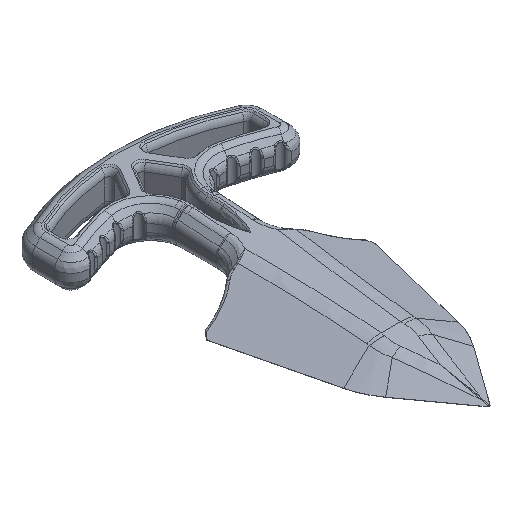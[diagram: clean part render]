
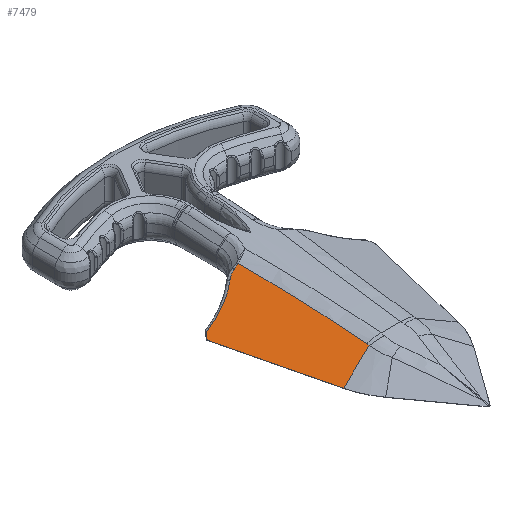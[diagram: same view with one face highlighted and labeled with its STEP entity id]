
A CAD part, isometric view. The second image highlights one B-rep face of the part: STEP entity #7479.
In plain terms, the highlighted planar face has unit normal (-0.411, -0.1, 0.906).
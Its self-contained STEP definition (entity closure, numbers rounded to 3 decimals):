
#197=PLANE('',#8067);
#256=ELLIPSE('',#8011,19.241,17.438);
#259=ELLIPSE('',#8065,2708.454,1112.419);
#261=ELLIPSE('',#8068,0.552,0.5);
#262=ELLIPSE('',#8069,4376.097,1797.354);
#309=LINE('',#11910,#611);
#310=LINE('',#11914,#612);
#311=LINE('',#11916,#613);
#611=VECTOR('',#9051,10.);
#612=VECTOR('',#9054,10.);
#613=VECTOR('',#9055,10.);
#1027=FACE_OUTER_BOUND('',#1552,.T.);
#1552=EDGE_LOOP('',(#5043,#5044,#5045,#5046,#5047,#5048,#5049,#5050,#5051));
#2093=B_SPLINE_CURVE_WITH_KNOTS('',3,(#11827,#11828,#11829,#11830),
 .UNSPECIFIED.,.F.,.F.,(4,4),(0.,0.131),.UNSPECIFIED.);
#2095=B_SPLINE_CURVE_WITH_KNOTS('',3,(#11861,#11862,#11863,#11864,#11865),
 .UNSPECIFIED.,.F.,.F.,(4,1,4),(0.,0.094,0.219),
 .UNSPECIFIED.);
#2963=VERTEX_POINT('',#11195);
#2964=VERTEX_POINT('',#11218);
#3048=VERTEX_POINT('',#11794);
#3050=VERTEX_POINT('',#11825);
#3051=VERTEX_POINT('',#11882);
#3053=VERTEX_POINT('',#11909);
#3054=VERTEX_POINT('',#11911);
#3055=VERTEX_POINT('',#11913);
#3056=VERTEX_POINT('',#11915);
#3673=EDGE_CURVE('',#2963,#2964,#256,.T.);
#3776=EDGE_CURVE('',#3050,#3048,#2093,.T.);
#3778=EDGE_CURVE('',#2964,#3050,#2095,.T.);
#3779=EDGE_CURVE('',#3048,#3051,#259,.T.);
#3782=EDGE_CURVE('',#3053,#2963,#309,.T.);
#3783=EDGE_CURVE('',#3054,#3053,#261,.T.);
#3784=EDGE_CURVE('',#3054,#3055,#310,.T.);
#3785=EDGE_CURVE('',#3055,#3056,#311,.T.);
#3786=EDGE_CURVE('',#3051,#3056,#262,.T.);
#5043=ORIENTED_EDGE('',*,*,#3776,.F.);
#5044=ORIENTED_EDGE('',*,*,#3778,.F.);
#5045=ORIENTED_EDGE('',*,*,#3673,.F.);
#5046=ORIENTED_EDGE('',*,*,#3782,.F.);
#5047=ORIENTED_EDGE('',*,*,#3783,.F.);
#5048=ORIENTED_EDGE('',*,*,#3784,.T.);
#5049=ORIENTED_EDGE('',*,*,#3785,.T.);
#5050=ORIENTED_EDGE('',*,*,#3786,.F.);
#5051=ORIENTED_EDGE('',*,*,#3779,.F.);
#7479=ADVANCED_FACE('',(#1027),#197,.T.);
#8011=AXIS2_PLACEMENT_3D('',#11219,#8913,#8914);
#8065=AXIS2_PLACEMENT_3D('',#11883,#9045,#9046);
#8067=AXIS2_PLACEMENT_3D('',#11908,#9049,#9050);
#8068=AXIS2_PLACEMENT_3D('',#11912,#9052,#9053);
#8069=AXIS2_PLACEMENT_3D('',#11917,#9056,#9057);
#8913=DIRECTION('center_axis',(-0.411,-0.1,0.906));
#8914=DIRECTION('ref_axis',(0.881,0.214,0.423));
#9045=DIRECTION('center_axis',(0.411,0.1,-0.906));
#9046=DIRECTION('ref_axis',(0.912,-0.045,0.408));
#9049=DIRECTION('center_axis',(-0.411,-0.1,0.906));
#9050=DIRECTION('ref_axis',(0.911,0.,0.413));
#9051=DIRECTION('',(0.569,0.749,0.34));
#9052=DIRECTION('center_axis',(0.411,0.1,-0.906));
#9053=DIRECTION('ref_axis',(-0.881,-0.214,-0.423));
#9054=DIRECTION('',(0.236,-0.972,0.));
#9055=DIRECTION('',(0.881,0.214,0.423));
#9056=DIRECTION('center_axis',(0.411,0.1,-0.906));
#9057=DIRECTION('ref_axis',(0.912,-0.045,0.408));
#11195=CARTESIAN_POINT('',(-19.524,-38.312,1.025));
#11218=CARTESIAN_POINT('',(-10.098,-34.726,5.691));
#11219=CARTESIAN_POINT('Origin',(-20.745,-20.916,2.383));
#11794=CARTESIAN_POINT('',(-7.126,-33.744,7.145));
#11825=CARTESIAN_POINT('',(-8.295,-33.924,6.596));
#11827=CARTESIAN_POINT('Ctrl Pts',(-8.295,-33.924,
6.596));
#11828=CARTESIAN_POINT('Ctrl Pts',(-7.901,-33.891,
6.778));
#11829=CARTESIAN_POINT('Ctrl Pts',(-7.51,-33.831,
6.962));
#11830=CARTESIAN_POINT('Ctrl Pts',(-7.126,-33.744,
7.145));
#11861=CARTESIAN_POINT('Ctrl Pts',(-10.098,-34.726,
5.691));
#11862=CARTESIAN_POINT('Ctrl Pts',(-9.87,-34.55,5.813));
#11863=CARTESIAN_POINT('Ctrl Pts',(-9.305,-34.192,
6.109));
#11864=CARTESIAN_POINT('Ctrl Pts',(-8.673,-33.955,
6.421));
#11865=CARTESIAN_POINT('Ctrl Pts',(-8.295,-33.924,
6.596));
#11882=CARTESIAN_POINT('',(-5.699,-63.574,4.515));
#11883=CARTESIAN_POINT('Origin',(-2475.083,49.058,-1102.187));
#11908=CARTESIAN_POINT('Origin',(-9.421,-46.079,4.75));
#11909=CARTESIAN_POINT('',(-20.258,-39.278,0.586));
#11910=CARTESIAN_POINT('',(-18.463,-36.915,1.659));
#11911=CARTESIAN_POINT('',(-20.346,-39.699,0.5));
#11912=CARTESIAN_POINT('Origin',(-19.86,-39.581,0.733));
#11913=CARTESIAN_POINT('',(-13.925,-66.185,0.5));
#11914=CARTESIAN_POINT('',(-18.279,-48.227,0.5));
#11915=CARTESIAN_POINT('',(-5.767,-64.207,4.414));
#11916=CARTESIAN_POINT('',(-13.925,-66.185,0.5));
#11917=CARTESIAN_POINT('Origin',(-3991.095,217.872,-1770.667));
